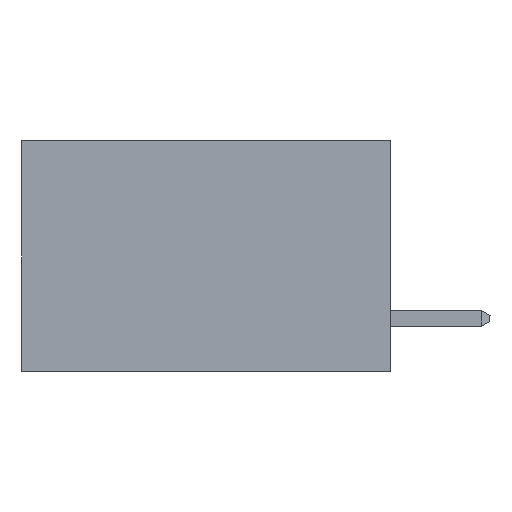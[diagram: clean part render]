
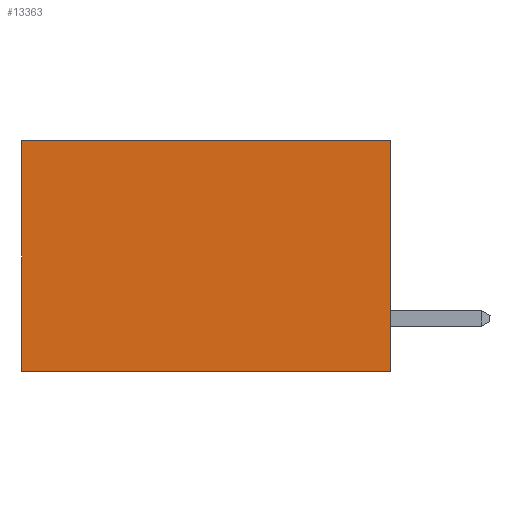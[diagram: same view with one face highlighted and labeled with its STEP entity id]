
A CAD part, left-side view. The second image highlights one B-rep face of the part: STEP entity #13363.
In plain terms, the highlighted planar face has unit normal (-1, 0, 0).
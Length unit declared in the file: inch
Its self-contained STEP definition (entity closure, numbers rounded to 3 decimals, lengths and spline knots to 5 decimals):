
#237 = LINE ( 'NONE', #948, #13675 ) ;
#355 = DIRECTION ( 'NONE',  ( 0., 1., 0. ) ) ;
#643 = DIRECTION ( 'NONE',  ( 0., 0., -1. ) ) ;
#661 = EDGE_CURVE ( 'NONE', #3032, #10116, #10906, .T. ) ;
#751 = DIRECTION ( 'NONE',  ( 0., 1., 0. ) ) ;
#948 = CARTESIAN_POINT ( 'NONE',  ( 0.277, 0., 0. ) ) ;
#1635 = VERTEX_POINT ( 'NONE', #13599 ) ;
#2223 = VECTOR ( 'NONE', #10805, 39.37008 ) ;
#2853 = AXIS2_PLACEMENT_3D ( 'NONE', #11533, #7257, #643 ) ;
#3032 = VERTEX_POINT ( 'NONE', #11515 ) ;
#4589 = CARTESIAN_POINT ( 'NONE',  ( 0.277, 0., -0.37 ) ) ;
#4727 = DIRECTION ( 'NONE',  ( 0., 0., -1. ) ) ;
#5883 = CARTESIAN_POINT ( 'NONE',  ( 0.277, 0., -0.37 ) ) ;
#6344 = EDGE_CURVE ( 'NONE', #1635, #3032, #237, .T. ) ;
#6868 = EDGE_CURVE ( 'NONE', #1635, #12986, #10201, .T. ) ;
#7257 = DIRECTION ( 'NONE',  ( 1., 0., 0. ) ) ;
#7762 = ORIENTED_EDGE ( 'NONE', *, *, #661, .T. ) ;
#8078 = ORIENTED_EDGE ( 'NONE', *, *, #6868, .F. ) ;
#8532 = CARTESIAN_POINT ( 'NONE',  ( 0.277, 0.59, -0.37 ) ) ;
#8585 = CARTESIAN_POINT ( 'NONE',  ( 0.277, 0.59, -0.37 ) ) ;
#9010 = EDGE_CURVE ( 'NONE', #12986, #10116, #13171, .T. ) ;
#9866 = VECTOR ( 'NONE', #4727, 39.37008 ) ;
#10116 = VERTEX_POINT ( 'NONE', #8532 ) ;
#10201 = LINE ( 'NONE', #4589, #9866 ) ;
#10372 = VECTOR ( 'NONE', #355, 39.37008 ) ;
#10620 = ORIENTED_EDGE ( 'NONE', *, *, #9010, .F. ) ;
#10805 = DIRECTION ( 'NONE',  ( 0., 0., -1. ) ) ;
#10906 = LINE ( 'NONE', #8585, #2223 ) ;
#10935 = ORIENTED_EDGE ( 'NONE', *, *, #6344, .T. ) ;
#11148 = FACE_OUTER_BOUND ( 'NONE', #13607, .T. ) ;
#11515 = CARTESIAN_POINT ( 'NONE',  ( 0.277, 0.59, 0. ) ) ;
#11533 = CARTESIAN_POINT ( 'NONE',  ( 0.277, 0., -0.37 ) ) ;
#12765 = CARTESIAN_POINT ( 'NONE',  ( 0.277, 0., -0.37 ) ) ;
#12986 = VERTEX_POINT ( 'NONE', #12765 ) ;
#13171 = LINE ( 'NONE', #5883, #10372 ) ;
#13363 = ADVANCED_FACE ( 'NONE', ( #11148 ), #13627, .F. ) ;
#13599 = CARTESIAN_POINT ( 'NONE',  ( 0.277, 0., 0. ) ) ;
#13607 = EDGE_LOOP ( 'NONE', ( #7762, #10620, #8078, #10935 ) ) ;
#13627 = PLANE ( 'NONE',  #2853 ) ;
#13675 = VECTOR ( 'NONE', #751, 39.37008 ) ;
